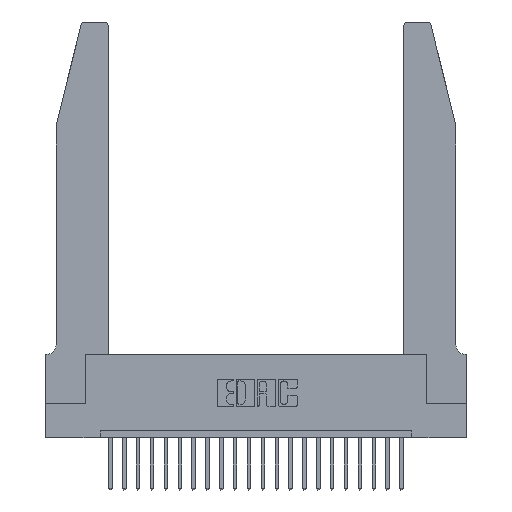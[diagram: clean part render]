
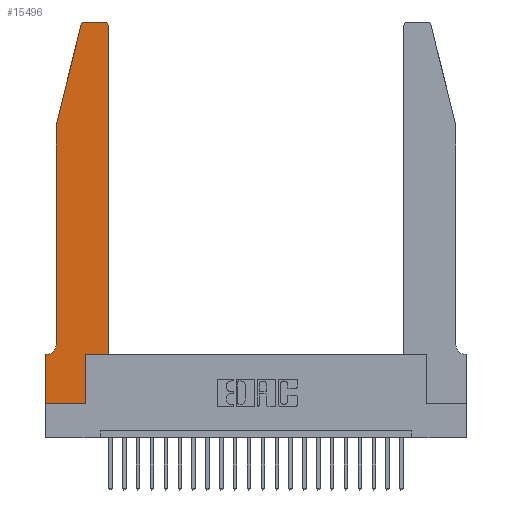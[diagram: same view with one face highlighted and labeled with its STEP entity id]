
A CAD part, top view. The second image highlights one B-rep face of the part: STEP entity #15496.
In plain terms, the highlighted planar face has unit normal (0, 0, 1).
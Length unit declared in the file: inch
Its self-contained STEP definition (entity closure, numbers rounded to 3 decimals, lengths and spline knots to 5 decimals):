
#101 = DIRECTION ( 'NONE',  ( -1., 0., 0. ) ) ;
#458 = DIRECTION ( 'NONE',  ( -0.239, -0.971, 0. ) ) ;
#942 = VECTOR ( 'NONE', #16870, 39.37008 ) ;
#1211 = DIRECTION ( 'NONE',  ( 0., 0., 1. ) ) ;
#1212 = EDGE_CURVE ( 'NONE', #23112, #18226, #2404, .T. ) ;
#2404 = LINE ( 'NONE', #2877, #6749 ) ;
#2800 = CARTESIAN_POINT ( 'NONE',  ( 0.0755, 2., 0.37 ) ) ;
#2877 = CARTESIAN_POINT ( 'NONE',  ( 0.2605, 2.75, 0.37 ) ) ;
#2896 = CARTESIAN_POINT ( 'NONE',  ( 0.284, 2.72, 0.37 ) ) ;
#2911 = AXIS2_PLACEMENT_3D ( 'NONE', #19826, #2936, #19982 ) ;
#2936 = DIRECTION ( 'NONE',  ( 0., 0., -1. ) ) ;
#3421 = CARTESIAN_POINT ( 'NONE',  ( 0.0055, 0.35, 0.37 ) ) ;
#3785 = LINE ( 'NONE', #15314, #21228 ) ;
#3853 = VECTOR ( 'NONE', #101, 39.37008 ) ;
#3895 = EDGE_CURVE ( 'NONE', #5850, #18808, #16477, .T. ) ;
#4200 = PLANE ( 'NONE',  #18214 ) ;
#4248 = VECTOR ( 'NONE', #13664, 39.37008 ) ;
#4458 = LINE ( 'NONE', #7535, #3853 ) ;
#4475 = CARTESIAN_POINT ( 'NONE',  ( 0.4505, 0.35, 0.37 ) ) ;
#4578 = ORIENTED_EDGE ( 'NONE', *, *, #17189, .T. ) ;
#4919 = EDGE_CURVE ( 'NONE', #5336, #17091, #4458, .T. ) ;
#5049 = VECTOR ( 'NONE', #5204, 39.37008 ) ;
#5204 = DIRECTION ( 'NONE',  ( 1., 0., 0. ) ) ;
#5278 = EDGE_CURVE ( 'NONE', #6303, #6814, #14489, .T. ) ;
#5336 = VERTEX_POINT ( 'NONE', #3421 ) ;
#5574 = ORIENTED_EDGE ( 'NONE', *, *, #11076, .T. ) ;
#5850 = VERTEX_POINT ( 'NONE', #20075 ) ;
#6267 = ORIENTED_EDGE ( 'NONE', *, *, #4919, .T. ) ;
#6303 = VERTEX_POINT ( 'NONE', #14100 ) ;
#6607 = AXIS2_PLACEMENT_3D ( 'NONE', #2896, #1211, #23251 ) ;
#6749 = VECTOR ( 'NONE', #15912, 39.37008 ) ;
#6814 = VERTEX_POINT ( 'NONE', #14755 ) ;
#6828 = DIRECTION ( 'NONE',  ( 1., 0., 0. ) ) ;
#7535 = CARTESIAN_POINT ( 'NONE',  ( 0.0755, 0.35, 0.37 ) ) ;
#8300 = DIRECTION ( 'NONE',  ( 0., 1., 0. ) ) ;
#9287 = DIRECTION ( 'NONE',  ( 0., 1., 0. ) ) ;
#9355 = CARTESIAN_POINT ( 'NONE',  ( 0.4205, 2.72, 0.37 ) ) ;
#9387 = CIRCLE ( 'NONE', #6607, 0.03 ) ;
#9645 = ORIENTED_EDGE ( 'NONE', *, *, #1212, .T. ) ;
#9709 = CARTESIAN_POINT ( 'NONE',  ( 0.0755, 0.42, 0.37 ) ) ;
#9897 = ORIENTED_EDGE ( 'NONE', *, *, #11767, .T. ) ;
#10156 = CIRCLE ( 'NONE', #23188, 0.03 ) ;
#10412 = DIRECTION ( 'NONE',  ( 1., 0., 0. ) ) ;
#11076 = EDGE_CURVE ( 'NONE', #17091, #17976, #12478, .T. ) ;
#11079 = CARTESIAN_POINT ( 'NONE',  ( 0., 0., 0.37 ) ) ;
#11098 = CARTESIAN_POINT ( 'NONE',  ( 0.284, 2.75, 0.37 ) ) ;
#11619 = EDGE_CURVE ( 'NONE', #22258, #23112, #10156, .T. ) ;
#11767 = EDGE_CURVE ( 'NONE', #17976, #5850, #15480, .T. ) ;
#11809 = CARTESIAN_POINT ( 'NONE',  ( 0., 0.35, 0.37 ) ) ;
#12083 = LINE ( 'NONE', #2800, #4248 ) ;
#12146 = DIRECTION ( 'NONE',  ( 0., 0., 1. ) ) ;
#12277 = VECTOR ( 'NONE', #6828, 39.37008 ) ;
#12376 = DIRECTION ( 'NONE',  ( 1., 0., 0. ) ) ;
#12478 = LINE ( 'NONE', #12796, #942 ) ;
#12519 = VERTEX_POINT ( 'NONE', #9709 ) ;
#12796 = CARTESIAN_POINT ( 'NONE',  ( 0., 0., 0.37 ) ) ;
#12975 = EDGE_CURVE ( 'NONE', #18907, #22258, #3785, .T. ) ;
#12981 = CARTESIAN_POINT ( 'NONE',  ( 0.2865, 0.35, 0.37 ) ) ;
#13369 = ORIENTED_EDGE ( 'NONE', *, *, #12975, .T. ) ;
#13608 = CARTESIAN_POINT ( 'NONE',  ( 0., 0.35, 0.37 ) ) ;
#13664 = DIRECTION ( 'NONE',  ( 0., -1., 0. ) ) ;
#14100 = CARTESIAN_POINT ( 'NONE',  ( 0.25487, 2.72718, 0.37 ) ) ;
#14171 = VECTOR ( 'NONE', #9287, 39.37008 ) ;
#14489 = LINE ( 'NONE', #22662, #20050 ) ;
#14755 = CARTESIAN_POINT ( 'NONE',  ( 0.0755, 2., 0.37 ) ) ;
#15314 = CARTESIAN_POINT ( 'NONE',  ( 0.4505, 0.35, 0.37 ) ) ;
#15480 = LINE ( 'NONE', #11079, #5049 ) ;
#15496 = ADVANCED_FACE ( 'NONE', ( #22603 ), #4200, .T. ) ;
#15694 = EDGE_LOOP ( 'NONE', ( #9645, #4578, #20375, #17158, #19797, #6267, #5574, #9897, #20256, #19335, #13369, #19615 ) ) ;
#15912 = DIRECTION ( 'NONE',  ( -1., 0., 0. ) ) ;
#16285 = CARTESIAN_POINT ( 'NONE',  ( 0., 0., 0.37 ) ) ;
#16477 = LINE ( 'NONE', #12981, #14171 ) ;
#16551 = CARTESIAN_POINT ( 'NONE',  ( 0.4205, 2.75, 0.37 ) ) ;
#16870 = DIRECTION ( 'NONE',  ( 0., -1., 0. ) ) ;
#17091 = VERTEX_POINT ( 'NONE', #13608 ) ;
#17158 = ORIENTED_EDGE ( 'NONE', *, *, #20064, .T. ) ;
#17189 = EDGE_CURVE ( 'NONE', #18226, #6303, #9387, .T. ) ;
#17976 = VERTEX_POINT ( 'NONE', #16285 ) ;
#18214 = AXIS2_PLACEMENT_3D ( 'NONE', #11809, #23021, #10412 ) ;
#18224 = CARTESIAN_POINT ( 'NONE',  ( 0.4505, 2.72, 0.37 ) ) ;
#18226 = VERTEX_POINT ( 'NONE', #11098 ) ;
#18808 = VERTEX_POINT ( 'NONE', #22563 ) ;
#18907 = VERTEX_POINT ( 'NONE', #22220 ) ;
#19335 = ORIENTED_EDGE ( 'NONE', *, *, #21610, .T. ) ;
#19615 = ORIENTED_EDGE ( 'NONE', *, *, #11619, .T. ) ;
#19797 = ORIENTED_EDGE ( 'NONE', *, *, #20719, .T. ) ;
#19826 = CARTESIAN_POINT ( 'NONE',  ( 0.0055, 0.42, 0.37 ) ) ;
#19982 = DIRECTION ( 'NONE',  ( -1., 0., 0. ) ) ;
#20050 = VECTOR ( 'NONE', #458, 39.37008 ) ;
#20064 = EDGE_CURVE ( 'NONE', #6814, #12519, #12083, .T. ) ;
#20075 = CARTESIAN_POINT ( 'NONE',  ( 0.2865, 0., 0.37 ) ) ;
#20256 = ORIENTED_EDGE ( 'NONE', *, *, #3895, .T. ) ;
#20375 = ORIENTED_EDGE ( 'NONE', *, *, #5278, .T. ) ;
#20505 = CIRCLE ( 'NONE', #2911, 0.07 ) ;
#20719 = EDGE_CURVE ( 'NONE', #12519, #5336, #20505, .T. ) ;
#21228 = VECTOR ( 'NONE', #8300, 39.37008 ) ;
#21610 = EDGE_CURVE ( 'NONE', #18808, #18907, #22149, .T. ) ;
#22149 = LINE ( 'NONE', #4475, #12277 ) ;
#22220 = CARTESIAN_POINT ( 'NONE',  ( 0.4505, 0.35, 0.37 ) ) ;
#22258 = VERTEX_POINT ( 'NONE', #18224 ) ;
#22563 = CARTESIAN_POINT ( 'NONE',  ( 0.2865, 0.35, 0.37 ) ) ;
#22603 = FACE_OUTER_BOUND ( 'NONE', #15694, .T. ) ;
#22662 = CARTESIAN_POINT ( 'NONE',  ( 0.0755, 2., 0.37 ) ) ;
#23021 = DIRECTION ( 'NONE',  ( 0., 0., 1. ) ) ;
#23112 = VERTEX_POINT ( 'NONE', #16551 ) ;
#23188 = AXIS2_PLACEMENT_3D ( 'NONE', #9355, #12146, #12376 ) ;
#23251 = DIRECTION ( 'NONE',  ( 1., 0., 0. ) ) ;
